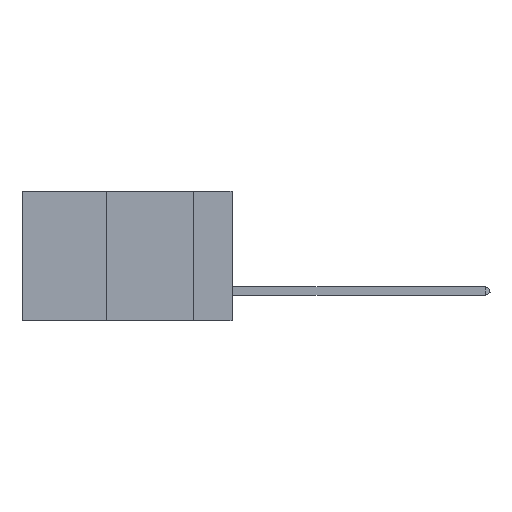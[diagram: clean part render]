
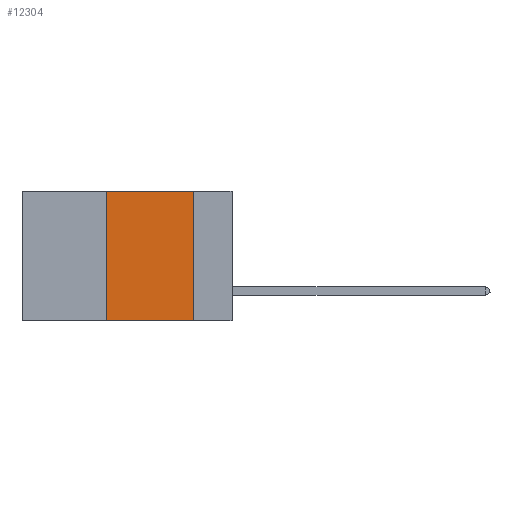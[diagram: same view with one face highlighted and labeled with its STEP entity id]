
A CAD part, left-side view. The second image highlights one B-rep face of the part: STEP entity #12304.
In plain terms, the highlighted planar face has unit normal (-1, 0, 0).
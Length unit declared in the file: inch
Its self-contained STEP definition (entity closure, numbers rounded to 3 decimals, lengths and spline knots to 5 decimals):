
#126 = VECTOR ( 'NONE', #1209, 39.37008 ) ;
#191 = CARTESIAN_POINT ( 'NONE',  ( 0., 0.36, -0.37 ) ) ;
#1209 = DIRECTION ( 'NONE',  ( 0., 0., 1. ) ) ;
#1453 = CARTESIAN_POINT ( 'NONE',  ( 0., 0.36, 0. ) ) ;
#1541 = DIRECTION ( 'NONE',  ( 0., -1., 0. ) ) ;
#1777 = VECTOR ( 'NONE', #11892, 39.37008 ) ;
#1966 = LINE ( 'NONE', #2607, #7356 ) ;
#2607 = CARTESIAN_POINT ( 'NONE',  ( 0., 0.6, 0. ) ) ;
#2678 = FACE_OUTER_BOUND ( 'NONE', #5259, .T. ) ;
#3192 = ORIENTED_EDGE ( 'NONE', *, *, #7124, .F. ) ;
#3419 = VERTEX_POINT ( 'NONE', #191 ) ;
#4241 = CARTESIAN_POINT ( 'NONE',  ( 0., 0.11, -0.37 ) ) ;
#4580 = EDGE_CURVE ( 'NONE', #5939, #7375, #1966, .T. ) ;
#4894 = EDGE_CURVE ( 'NONE', #7375, #12660, #5363, .T. ) ;
#5259 = EDGE_LOOP ( 'NONE', ( #9681, #6031, #3192, #10285 ) ) ;
#5363 = LINE ( 'NONE', #8290, #1777 ) ;
#5450 = AXIS2_PLACEMENT_3D ( 'NONE', #7053, #13033, #11823 ) ;
#5939 = VERTEX_POINT ( 'NONE', #10510 ) ;
#6031 = ORIENTED_EDGE ( 'NONE', *, *, #4580, .F. ) ;
#6258 = CARTESIAN_POINT ( 'NONE',  ( 0., 0.11, 0. ) ) ;
#7053 = CARTESIAN_POINT ( 'NONE',  ( 0., 0.6, 0. ) ) ;
#7124 = EDGE_CURVE ( 'NONE', #3419, #5939, #14824, .T. ) ;
#7356 = VECTOR ( 'NONE', #1541, 39.37008 ) ;
#7375 = VERTEX_POINT ( 'NONE', #6258 ) ;
#8290 = CARTESIAN_POINT ( 'NONE',  ( 0., 0.11, 0. ) ) ;
#9157 = EDGE_CURVE ( 'NONE', #3419, #12660, #14951, .T. ) ;
#9681 = ORIENTED_EDGE ( 'NONE', *, *, #4894, .F. ) ;
#10108 = CARTESIAN_POINT ( 'NONE',  ( 0., 0.6, -0.37 ) ) ;
#10285 = ORIENTED_EDGE ( 'NONE', *, *, #9157, .T. ) ;
#10510 = CARTESIAN_POINT ( 'NONE',  ( 0., 0.36, 0. ) ) ;
#10765 = VECTOR ( 'NONE', #12396, 39.37008 ) ;
#11823 = DIRECTION ( 'NONE',  ( 0., 0., -1. ) ) ;
#11892 = DIRECTION ( 'NONE',  ( 0., 0., -1. ) ) ;
#12304 = ADVANCED_FACE ( 'NONE', ( #2678 ), #14075, .F. ) ;
#12396 = DIRECTION ( 'NONE',  ( 0., -1., 0. ) ) ;
#12660 = VERTEX_POINT ( 'NONE', #4241 ) ;
#13033 = DIRECTION ( 'NONE',  ( 1., 0., 0. ) ) ;
#14075 = PLANE ( 'NONE',  #5450 ) ;
#14824 = LINE ( 'NONE', #1453, #126 ) ;
#14951 = LINE ( 'NONE', #10108, #10765 ) ;
